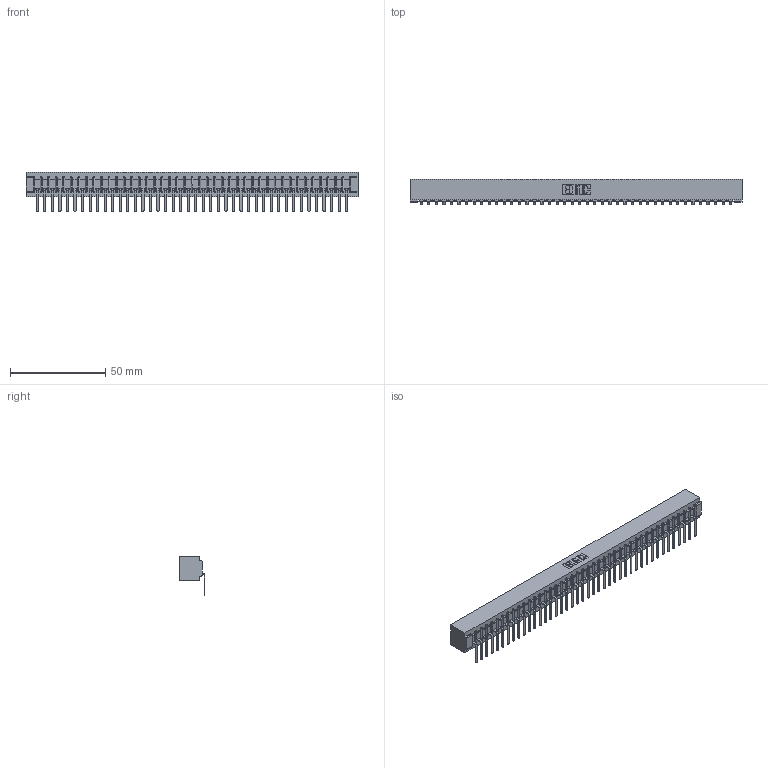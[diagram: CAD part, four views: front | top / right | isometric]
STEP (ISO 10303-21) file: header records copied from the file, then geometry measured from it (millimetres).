
FILE_DESCRIPTION (( 'STEP AP203' ), '1' );
FILE_NAME ('357-042-557-101.STEP', '2019-09-17T10:38:56', ( '' ), ( '' ), 'SwSTEP 2.0', 'SolidWorks 2016', '' );
FILE_SCHEMA (( 'CONFIG_CONTROL_DESIGN' ));
Length unit declared in the file: inch
Products named in the file (3): 307-290-002_557; 357-042-557-101; 307 Part_No Mounting Lugs
Assembly tree (43 placements, depth 2):
  357-042-557-101
    307 Part_No Mounting Lugs
    307-290-002_557  x42
Bounding box: 174.29 x 13.32 x 20.66 mm (x, y, z)
Volume: 19322.8 mm3; surface area: 25382 mm2
Topology: 43 solids, 43 shells, 3429 faces, 10547 edges, 6914 vertices
Faces by surface type: plane 2040, cylinder 1303, sphere 86
Entity records: 36582 total; most frequent: CARTESIAN_POINT 6172, ORIENTED_EDGE 6162, DIRECTION 5995, EDGE_CURVE 3081, VECTOR 2361, LINE 2361, VERTEX_POINT 1994, AXIS2_PLACEMENT_3D 1817
